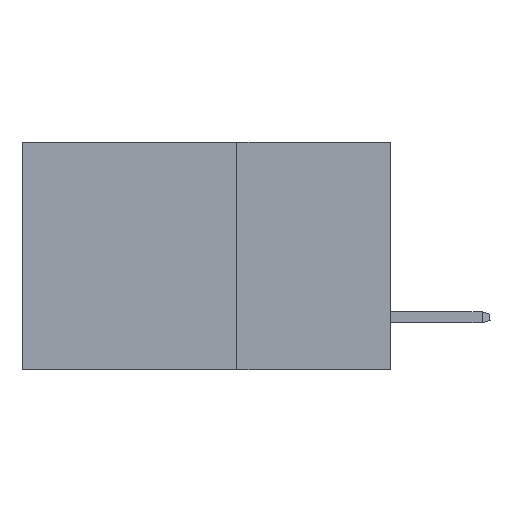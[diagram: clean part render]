
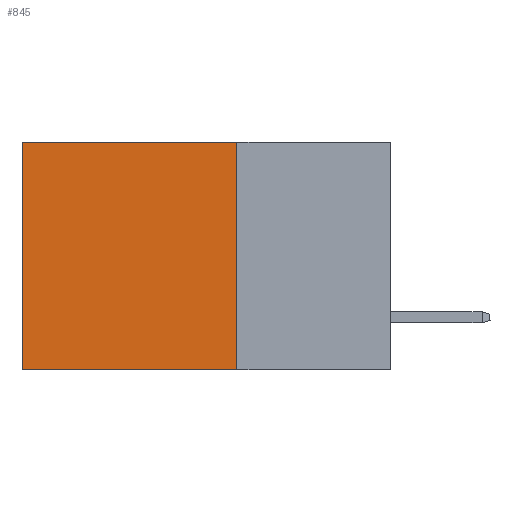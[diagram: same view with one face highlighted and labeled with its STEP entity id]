
A CAD part, left-side view. The second image highlights one B-rep face of the part: STEP entity #845.
In plain terms, the highlighted planar face has unit normal (-1, 0, 0).
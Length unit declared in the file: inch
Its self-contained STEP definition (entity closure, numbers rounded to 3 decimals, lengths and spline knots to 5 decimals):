
#309 = VERTEX_POINT ( 'NONE', #10572 ) ;
#603 = EDGE_CURVE ( 'NONE', #3469, #309, #6264, .T. ) ;
#845 = ADVANCED_FACE ( 'NONE', ( #5360 ), #17566, .F. ) ;
#2128 = DIRECTION ( 'NONE',  ( 0., 0., -1. ) ) ;
#2731 = EDGE_CURVE ( 'NONE', #24144, #12509, #9410, .T. ) ;
#3469 = VERTEX_POINT ( 'NONE', #19505 ) ;
#4406 = VECTOR ( 'NONE', #15478, 39.37008 ) ;
#4932 = CARTESIAN_POINT ( 'NONE',  ( 0.2875, 0.25, 0. ) ) ;
#5086 = DIRECTION ( 'NONE',  ( 0., 0., -1. ) ) ;
#5360 = FACE_OUTER_BOUND ( 'NONE', #23850, .T. ) ;
#6056 = CARTESIAN_POINT ( 'NONE',  ( 0.2875, 0.25, 0. ) ) ;
#6235 = ORIENTED_EDGE ( 'NONE', *, *, #21527, .T. ) ;
#6264 = LINE ( 'NONE', #4932, #15119 ) ;
#8431 = CARTESIAN_POINT ( 'NONE',  ( 0.2875, 0.6, 0. ) ) ;
#9410 = LINE ( 'NONE', #15277, #4406 ) ;
#10572 = CARTESIAN_POINT ( 'NONE',  ( 0.2875, 0.6, 0. ) ) ;
#12262 = DIRECTION ( 'NONE',  ( 0., 0., -1. ) ) ;
#12509 = VERTEX_POINT ( 'NONE', #15838 ) ;
#13657 = ORIENTED_EDGE ( 'NONE', *, *, #22783, .F. ) ;
#13937 = CARTESIAN_POINT ( 'NONE',  ( 0.2875, 0.25, -0.37 ) ) ;
#14888 = LINE ( 'NONE', #16428, #19233 ) ;
#15119 = VECTOR ( 'NONE', #18153, 39.37008 ) ;
#15277 = CARTESIAN_POINT ( 'NONE',  ( 0.2875, 0.25, -0.37 ) ) ;
#15478 = DIRECTION ( 'NONE',  ( 0., 1., 0. ) ) ;
#15496 = LINE ( 'NONE', #8431, #19788 ) ;
#15501 = ORIENTED_EDGE ( 'NONE', *, *, #603, .T. ) ;
#15690 = DIRECTION ( 'NONE',  ( 1., 0., 0. ) ) ;
#15838 = CARTESIAN_POINT ( 'NONE',  ( 0.2875, 0.6, -0.37 ) ) ;
#16428 = CARTESIAN_POINT ( 'NONE',  ( 0.2875, 0.25, 0. ) ) ;
#17566 = PLANE ( 'NONE',  #21025 ) ;
#18153 = DIRECTION ( 'NONE',  ( 0., 1., 0. ) ) ;
#18883 = ORIENTED_EDGE ( 'NONE', *, *, #2731, .F. ) ;
#19233 = VECTOR ( 'NONE', #5086, 39.37008 ) ;
#19505 = CARTESIAN_POINT ( 'NONE',  ( 0.2875, 0.25, 0. ) ) ;
#19788 = VECTOR ( 'NONE', #12262, 39.37008 ) ;
#21025 = AXIS2_PLACEMENT_3D ( 'NONE', #6056, #15690, #2128 ) ;
#21527 = EDGE_CURVE ( 'NONE', #309, #12509, #15496, .T. ) ;
#22783 = EDGE_CURVE ( 'NONE', #3469, #24144, #14888, .T. ) ;
#23850 = EDGE_LOOP ( 'NONE', ( #6235, #18883, #13657, #15501 ) ) ;
#24144 = VERTEX_POINT ( 'NONE', #13937 ) ;
